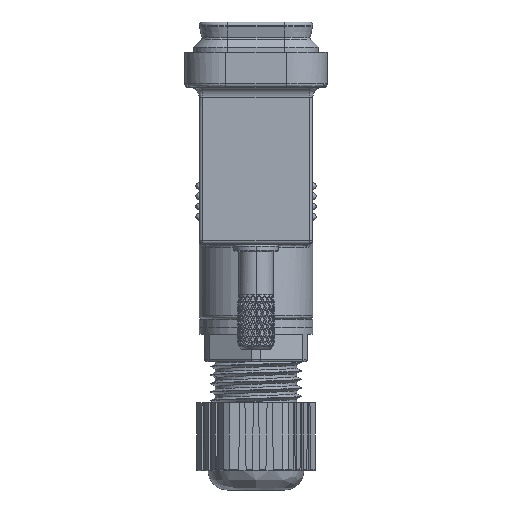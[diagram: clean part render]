
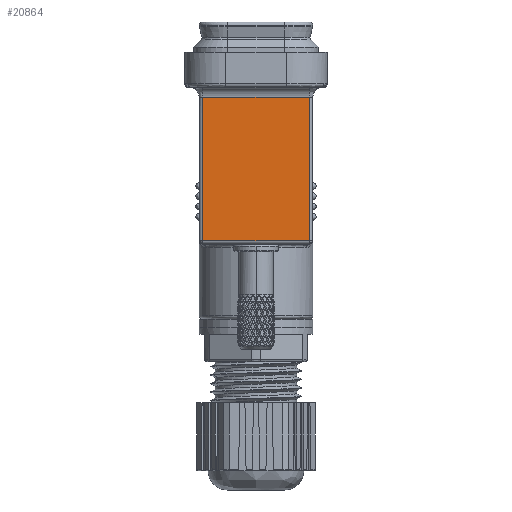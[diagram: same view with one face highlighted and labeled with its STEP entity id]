
A CAD part, front view. The second image highlights one B-rep face of the part: STEP entity #20864.
In plain terms, the highlighted planar face has unit normal (0, -1, 0).
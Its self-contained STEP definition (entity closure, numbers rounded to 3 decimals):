
#1616 = DIRECTION ( 'NONE',  ( 1., 0., 0. ) ) ;
#7062 = DIRECTION ( 'NONE',  ( 0., 0., 1. ) ) ;
#11501 = DIRECTION ( 'NONE',  ( 0., 0., 1. ) ) ;
#12629 = VERTEX_POINT ( 'NONE', #38014 ) ;
#14358 = VECTOR ( 'NONE', #83379, 1000. ) ;
#14528 = ORIENTED_EDGE ( 'NONE', *, *, #77655, .F. ) ;
#18532 = EDGE_CURVE ( 'NONE', #67850, #85859, #89745, .T. ) ;
#18918 = CARTESIAN_POINT ( 'NONE',  ( 10.45, -21.085, -32.31 ) ) ;
#20864 = ADVANCED_FACE ( 'NONE', ( #46221 ), #25719, .F. ) ;
#21435 = LINE ( 'NONE', #84256, #14358 ) ;
#25719 = PLANE ( 'NONE',  #60502 ) ;
#29654 = ORIENTED_EDGE ( 'NONE', *, *, #40243, .F. ) ;
#32436 = CARTESIAN_POINT ( 'NONE',  ( -7.8, -21.085, -32.31 ) ) ;
#34545 = LINE ( 'NONE', #75069, #49763 ) ;
#35812 = ORIENTED_EDGE ( 'NONE', *, *, #74877, .F. ) ;
#38014 = CARTESIAN_POINT ( 'NONE',  ( -7.8, -21.085, -6.65 ) ) ;
#40243 = EDGE_CURVE ( 'NONE', #12629, #57846, #34545, .T. ) ;
#46221 = FACE_OUTER_BOUND ( 'NONE', #59171, .T. ) ;
#47506 = VECTOR ( 'NONE', #76108, 1000. ) ;
#49763 = VECTOR ( 'NONE', #1616, 1000. ) ;
#54680 = CARTESIAN_POINT ( 'NONE',  ( 7.8, -21.085, -27.6 ) ) ;
#57521 = DIRECTION ( 'NONE',  ( 0., 1., 0. ) ) ;
#57846 = VERTEX_POINT ( 'NONE', #67976 ) ;
#59171 = EDGE_LOOP ( 'NONE', ( #62354, #14528, #29654, #35812 ) ) ;
#60502 = AXIS2_PLACEMENT_3D ( 'NONE', #18918, #57521, #7062 ) ;
#62354 = ORIENTED_EDGE ( 'NONE', *, *, #18532, .F. ) ;
#63322 = CARTESIAN_POINT ( 'NONE',  ( 10.45, -21.085, -27.6 ) ) ;
#67507 = LINE ( 'NONE', #32436, #72588 ) ;
#67850 = VERTEX_POINT ( 'NONE', #54680 ) ;
#67976 = CARTESIAN_POINT ( 'NONE',  ( 7.8, -21.085, -6.65 ) ) ;
#72588 = VECTOR ( 'NONE', #11501, 1000. ) ;
#74877 = EDGE_CURVE ( 'NONE', #85859, #12629, #67507, .T. ) ;
#75069 = CARTESIAN_POINT ( 'NONE',  ( 10.45, -21.085, -6.65 ) ) ;
#76108 = DIRECTION ( 'NONE',  ( -1., 0., 0. ) ) ;
#77655 = EDGE_CURVE ( 'NONE', #57846, #67850, #21435, .T. ) ;
#83379 = DIRECTION ( 'NONE',  ( 0., 0., -1. ) ) ;
#84256 = CARTESIAN_POINT ( 'NONE',  ( 7.8, -21.085, -5.041 ) ) ;
#85859 = VERTEX_POINT ( 'NONE', #85864 ) ;
#85864 = CARTESIAN_POINT ( 'NONE',  ( -7.8, -21.085, -27.6 ) ) ;
#89745 = LINE ( 'NONE', #63322, #47506 ) ;
